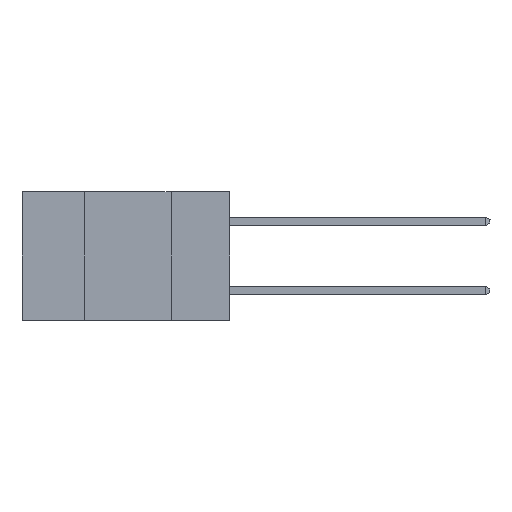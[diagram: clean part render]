
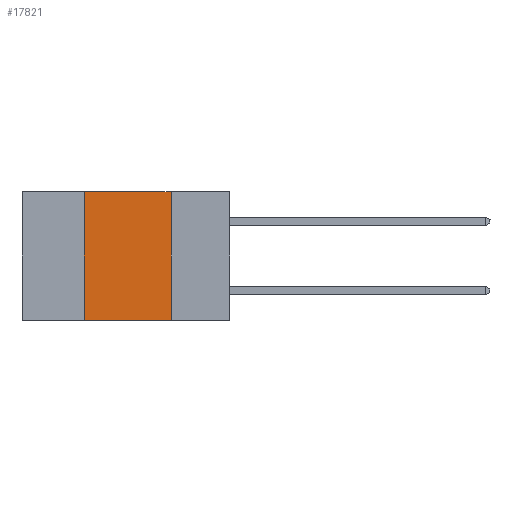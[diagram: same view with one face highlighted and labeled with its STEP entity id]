
A CAD part, left-side view. The second image highlights one B-rep face of the part: STEP entity #17821.
In plain terms, the highlighted planar face has unit normal (-1, 0, 0).
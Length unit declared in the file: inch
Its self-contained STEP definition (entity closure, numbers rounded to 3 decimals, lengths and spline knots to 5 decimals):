
#80 = EDGE_CURVE ( 'NONE', #16660, #16361, #8991, .T. ) ;
#518 = AXIS2_PLACEMENT_3D ( 'NONE', #17645, #8211, #19140 ) ;
#673 = CARTESIAN_POINT ( 'NONE',  ( 0., 0.17, 0. ) ) ;
#929 = VECTOR ( 'NONE', #18056, 39.37008 ) ;
#1325 = CARTESIAN_POINT ( 'NONE',  ( 0., 0.6, -0.37 ) ) ;
#2067 = EDGE_CURVE ( 'NONE', #16660, #17820, #12867, .T. ) ;
#2540 = VECTOR ( 'NONE', #14826, 39.37008 ) ;
#2767 = LINE ( 'NONE', #673, #7087 ) ;
#3658 = CARTESIAN_POINT ( 'NONE',  ( 0., 0.6, 0. ) ) ;
#3697 = ORIENTED_EDGE ( 'NONE', *, *, #80, .T. ) ;
#4291 = VERTEX_POINT ( 'NONE', #17748 ) ;
#4377 = VECTOR ( 'NONE', #14317, 39.37008 ) ;
#5416 = CARTESIAN_POINT ( 'NONE',  ( 0., 0.42, 0. ) ) ;
#6039 = CARTESIAN_POINT ( 'NONE',  ( 0., 0.17, -0.37 ) ) ;
#6625 = PLANE ( 'NONE',  #518 ) ;
#6808 = CARTESIAN_POINT ( 'NONE',  ( 0., 0.42, -0.37 ) ) ;
#7087 = VECTOR ( 'NONE', #16585, 39.37008 ) ;
#8211 = DIRECTION ( 'NONE',  ( 1., 0., 0. ) ) ;
#8991 = LINE ( 'NONE', #1325, #929 ) ;
#9764 = EDGE_LOOP ( 'NONE', ( #18532, #15430, #15921, #3697 ) ) ;
#10007 = EDGE_CURVE ( 'NONE', #4291, #16361, #2767, .T. ) ;
#11321 = CARTESIAN_POINT ( 'NONE',  ( 0., 0.42, 0. ) ) ;
#12867 = LINE ( 'NONE', #5416, #4377 ) ;
#14317 = DIRECTION ( 'NONE',  ( 0., 0., 1. ) ) ;
#14786 = LINE ( 'NONE', #3658, #2540 ) ;
#14826 = DIRECTION ( 'NONE',  ( 0., -1., 0. ) ) ;
#15430 = ORIENTED_EDGE ( 'NONE', *, *, #20184, .F. ) ;
#15921 = ORIENTED_EDGE ( 'NONE', *, *, #2067, .F. ) ;
#16123 = FACE_OUTER_BOUND ( 'NONE', #9764, .T. ) ;
#16361 = VERTEX_POINT ( 'NONE', #6039 ) ;
#16585 = DIRECTION ( 'NONE',  ( 0., 0., -1. ) ) ;
#16660 = VERTEX_POINT ( 'NONE', #6808 ) ;
#17645 = CARTESIAN_POINT ( 'NONE',  ( 0., 0.6, 0. ) ) ;
#17748 = CARTESIAN_POINT ( 'NONE',  ( 0., 0.17, 0. ) ) ;
#17820 = VERTEX_POINT ( 'NONE', #11321 ) ;
#17821 = ADVANCED_FACE ( 'NONE', ( #16123 ), #6625, .F. ) ;
#18056 = DIRECTION ( 'NONE',  ( 0., -1., 0. ) ) ;
#18532 = ORIENTED_EDGE ( 'NONE', *, *, #10007, .F. ) ;
#19140 = DIRECTION ( 'NONE',  ( 0., 0., -1. ) ) ;
#20184 = EDGE_CURVE ( 'NONE', #17820, #4291, #14786, .T. ) ;
